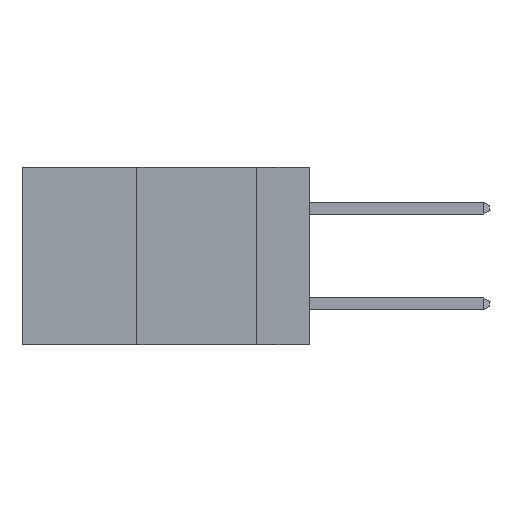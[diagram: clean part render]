
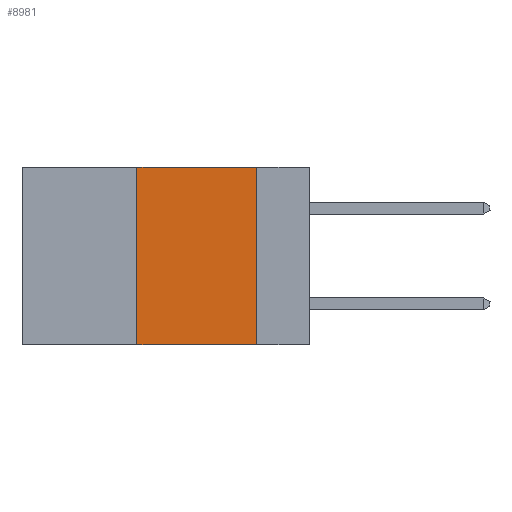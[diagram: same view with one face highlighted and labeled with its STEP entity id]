
A CAD part, left-side view. The second image highlights one B-rep face of the part: STEP entity #8981.
In plain terms, the highlighted planar face has unit normal (-1, 0, 0).
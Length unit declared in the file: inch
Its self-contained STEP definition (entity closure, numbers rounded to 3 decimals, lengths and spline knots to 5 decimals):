
#1421 = VECTOR ( 'NONE', #10239, 39.37008 ) ;
#3704 = LINE ( 'NONE', #5311, #9919 ) ;
#4242 = VERTEX_POINT ( 'NONE', #16118 ) ;
#5311 = CARTESIAN_POINT ( 'NONE',  ( 0., 0.6, 0. ) ) ;
#5725 = VECTOR ( 'NONE', #36615, 39.37008 ) ;
#6246 = EDGE_LOOP ( 'NONE', ( #15753, #11727, #17417, #14053 ) ) ;
#8909 = VERTEX_POINT ( 'NONE', #45188 ) ;
#8981 = ADVANCED_FACE ( 'NONE', ( #23581 ), #20764, .F. ) ;
#9919 = VECTOR ( 'NONE', #30652, 39.37008 ) ;
#10208 = VERTEX_POINT ( 'NONE', #26573 ) ;
#10239 = DIRECTION ( 'NONE',  ( 0., -1., 0. ) ) ;
#11727 = ORIENTED_EDGE ( 'NONE', *, *, #22245, .F. ) ;
#14053 = ORIENTED_EDGE ( 'NONE', *, *, #44583, .T. ) ;
#15543 = CARTESIAN_POINT ( 'NONE',  ( 0., 0.11, 0. ) ) ;
#15753 = ORIENTED_EDGE ( 'NONE', *, *, #19465, .F. ) ;
#16118 = CARTESIAN_POINT ( 'NONE',  ( 0., 0.36, -0.37 ) ) ;
#17417 = ORIENTED_EDGE ( 'NONE', *, *, #31607, .F. ) ;
#17474 = DIRECTION ( 'NONE',  ( 1., 0., 0. ) ) ;
#19465 = EDGE_CURVE ( 'NONE', #10208, #27440, #38292, .T. ) ;
#20764 = PLANE ( 'NONE',  #40479 ) ;
#21066 = DIRECTION ( 'NONE',  ( 0., 0., -1. ) ) ;
#22245 = EDGE_CURVE ( 'NONE', #8909, #10208, #3704, .T. ) ;
#23581 = FACE_OUTER_BOUND ( 'NONE', #6246, .T. ) ;
#26573 = CARTESIAN_POINT ( 'NONE',  ( 0., 0.11, 0. ) ) ;
#27440 = VERTEX_POINT ( 'NONE', #43296 ) ;
#28267 = LINE ( 'NONE', #36762, #5725 ) ;
#30652 = DIRECTION ( 'NONE',  ( 0., -1., 0. ) ) ;
#31607 = EDGE_CURVE ( 'NONE', #4242, #8909, #28267, .T. ) ;
#31811 = LINE ( 'NONE', #38410, #1421 ) ;
#36615 = DIRECTION ( 'NONE',  ( 0., 0., 1. ) ) ;
#36762 = CARTESIAN_POINT ( 'NONE',  ( 0., 0.36, 0. ) ) ;
#38292 = LINE ( 'NONE', #15543, #38841 ) ;
#38410 = CARTESIAN_POINT ( 'NONE',  ( 0., 0.6, -0.37 ) ) ;
#38841 = VECTOR ( 'NONE', #44323, 39.37008 ) ;
#40479 = AXIS2_PLACEMENT_3D ( 'NONE', #45957, #17474, #21066 ) ;
#43296 = CARTESIAN_POINT ( 'NONE',  ( 0., 0.11, -0.37 ) ) ;
#44323 = DIRECTION ( 'NONE',  ( 0., 0., -1. ) ) ;
#44583 = EDGE_CURVE ( 'NONE', #4242, #27440, #31811, .T. ) ;
#45188 = CARTESIAN_POINT ( 'NONE',  ( 0., 0.36, 0. ) ) ;
#45957 = CARTESIAN_POINT ( 'NONE',  ( 0., 0.6, 0. ) ) ;
